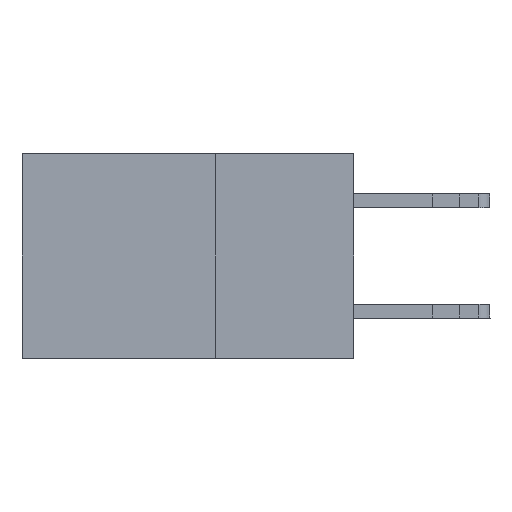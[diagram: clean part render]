
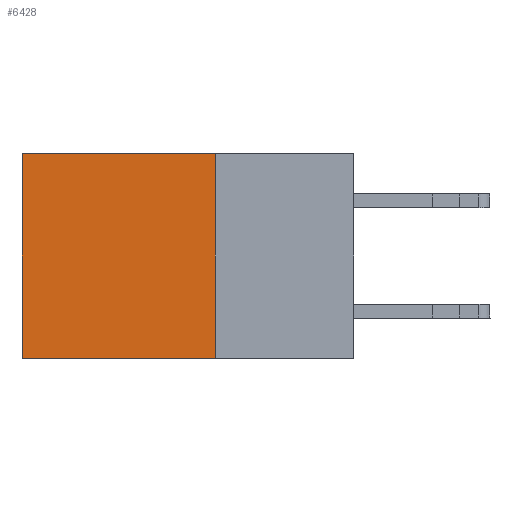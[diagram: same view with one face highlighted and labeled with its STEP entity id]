
A CAD part, left-side view. The second image highlights one B-rep face of the part: STEP entity #6428.
In plain terms, the highlighted planar face has unit normal (-1, 0, 0).
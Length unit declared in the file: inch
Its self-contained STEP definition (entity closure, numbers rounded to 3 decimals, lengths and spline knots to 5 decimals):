
#517 = DIRECTION ( 'NONE',  ( 1., 0., 0. ) ) ;
#1410 = ORIENTED_EDGE ( 'NONE', *, *, #16735, .T. ) ;
#1717 = VERTEX_POINT ( 'NONE', #13082 ) ;
#2048 = VERTEX_POINT ( 'NONE', #17692 ) ;
#2309 = EDGE_CURVE ( 'NONE', #1717, #30099, #4066, .T. ) ;
#4066 = LINE ( 'NONE', #26605, #11323 ) ;
#4358 = LINE ( 'NONE', #11724, #24387 ) ;
#5075 = PLANE ( 'NONE',  #15075 ) ;
#5278 = DIRECTION ( 'NONE',  ( 0., 0., -1. ) ) ;
#6428 = ADVANCED_FACE ( 'NONE', ( #20130 ), #5075, .F. ) ;
#7472 = CARTESIAN_POINT ( 'NONE',  ( 0.2875, 0.25, 0. ) ) ;
#9153 = LINE ( 'NONE', #10893, #22946 ) ;
#9650 = LINE ( 'NONE', #7472, #29975 ) ;
#10167 = ORIENTED_EDGE ( 'NONE', *, *, #28533, .T. ) ;
#10309 = CARTESIAN_POINT ( 'NONE',  ( 0.2875, 0.6, -0.37 ) ) ;
#10476 = CARTESIAN_POINT ( 'NONE',  ( 0.2875, 0.25, 0. ) ) ;
#10893 = CARTESIAN_POINT ( 'NONE',  ( 0.2875, 0.25, 0. ) ) ;
#11278 = VERTEX_POINT ( 'NONE', #10476 ) ;
#11323 = VECTOR ( 'NONE', #23947, 39.37008 ) ;
#11724 = CARTESIAN_POINT ( 'NONE',  ( 0.2875, 0.6, 0. ) ) ;
#13082 = CARTESIAN_POINT ( 'NONE',  ( 0.2875, 0.25, -0.37 ) ) ;
#13654 = DIRECTION ( 'NONE',  ( 0., 1., 0. ) ) ;
#15075 = AXIS2_PLACEMENT_3D ( 'NONE', #21322, #517, #5278 ) ;
#16735 = EDGE_CURVE ( 'NONE', #2048, #30099, #4358, .T. ) ;
#17692 = CARTESIAN_POINT ( 'NONE',  ( 0.2875, 0.6, 0. ) ) ;
#20130 = FACE_OUTER_BOUND ( 'NONE', #25871, .T. ) ;
#21322 = CARTESIAN_POINT ( 'NONE',  ( 0.2875, 0.25, 0. ) ) ;
#22946 = VECTOR ( 'NONE', #13654, 39.37008 ) ;
#23947 = DIRECTION ( 'NONE',  ( 0., 1., 0. ) ) ;
#24047 = ORIENTED_EDGE ( 'NONE', *, *, #2309, .F. ) ;
#24387 = VECTOR ( 'NONE', #25504, 39.37008 ) ;
#25504 = DIRECTION ( 'NONE',  ( 0., 0., -1. ) ) ;
#25871 = EDGE_LOOP ( 'NONE', ( #1410, #24047, #26799, #10167 ) ) ;
#26605 = CARTESIAN_POINT ( 'NONE',  ( 0.2875, 0.25, -0.37 ) ) ;
#26652 = EDGE_CURVE ( 'NONE', #11278, #1717, #9650, .T. ) ;
#26799 = ORIENTED_EDGE ( 'NONE', *, *, #26652, .F. ) ;
#28073 = DIRECTION ( 'NONE',  ( 0., 0., -1. ) ) ;
#28533 = EDGE_CURVE ( 'NONE', #11278, #2048, #9153, .T. ) ;
#29975 = VECTOR ( 'NONE', #28073, 39.37008 ) ;
#30099 = VERTEX_POINT ( 'NONE', #10309 ) ;
